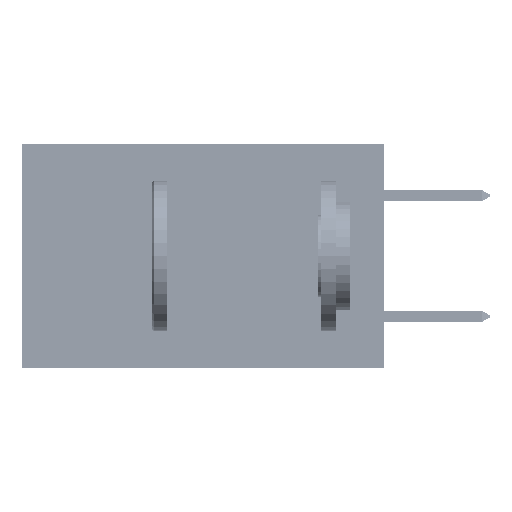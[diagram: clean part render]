
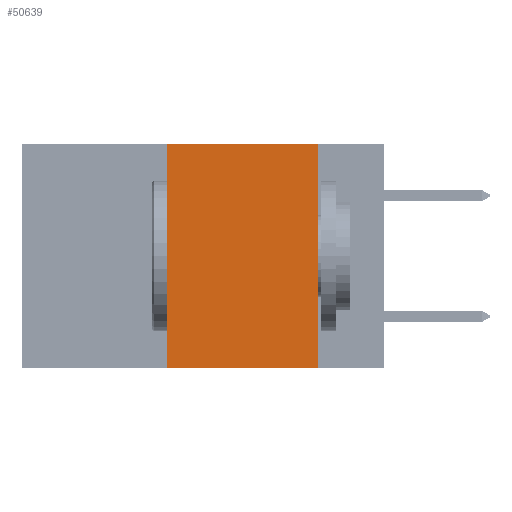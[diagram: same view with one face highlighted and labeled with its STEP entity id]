
A CAD part, left-side view. The second image highlights one B-rep face of the part: STEP entity #50639.
In plain terms, the highlighted planar face has unit normal (-1, 0, 0).
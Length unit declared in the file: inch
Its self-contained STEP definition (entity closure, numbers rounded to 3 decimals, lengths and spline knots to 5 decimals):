
#473 = VERTEX_POINT ( 'NONE', #18248 ) ;
#1398 = EDGE_LOOP ( 'NONE', ( #3842, #28397, #49163, #30030 ) ) ;
#3344 = VERTEX_POINT ( 'NONE', #49609 ) ;
#3842 = ORIENTED_EDGE ( 'NONE', *, *, #40647, .F. ) ;
#6336 = VECTOR ( 'NONE', #15519, 39.37008 ) ;
#7447 = LINE ( 'NONE', #50483, #43692 ) ;
#12015 = DIRECTION ( 'NONE',  ( 0., 0., -1. ) ) ;
#13848 = VERTEX_POINT ( 'NONE', #45142 ) ;
#13962 = AXIS2_PLACEMENT_3D ( 'NONE', #43008, #50385, #27043 ) ;
#15519 = DIRECTION ( 'NONE',  ( 0., -1., 0. ) ) ;
#17990 = LINE ( 'NONE', #35624, #6336 ) ;
#18248 = CARTESIAN_POINT ( 'NONE',  ( 0., 0.11, 0. ) ) ;
#19145 = PLANE ( 'NONE',  #13962 ) ;
#19431 = FACE_OUTER_BOUND ( 'NONE', #1398, .T. ) ;
#21513 = EDGE_CURVE ( 'NONE', #22364, #3344, #48150, .T. ) ;
#22288 = EDGE_CURVE ( 'NONE', #13848, #473, #17990, .T. ) ;
#22364 = VERTEX_POINT ( 'NONE', #38914 ) ;
#25880 = DIRECTION ( 'NONE',  ( 0., 0., 1. ) ) ;
#27043 = DIRECTION ( 'NONE',  ( 0., 0., -1. ) ) ;
#28397 = ORIENTED_EDGE ( 'NONE', *, *, #22288, .F. ) ;
#30030 = ORIENTED_EDGE ( 'NONE', *, *, #21513, .T. ) ;
#32541 = DIRECTION ( 'NONE',  ( 0., -1., 0. ) ) ;
#35624 = CARTESIAN_POINT ( 'NONE',  ( 0., 0.6, 0. ) ) ;
#35889 = EDGE_CURVE ( 'NONE', #22364, #13848, #7447, .T. ) ;
#37638 = LINE ( 'NONE', #43600, #43152 ) ;
#37717 = VECTOR ( 'NONE', #32541, 39.37008 ) ;
#38914 = CARTESIAN_POINT ( 'NONE',  ( 0., 0.36, -0.37 ) ) ;
#40647 = EDGE_CURVE ( 'NONE', #473, #3344, #37638, .T. ) ;
#43008 = CARTESIAN_POINT ( 'NONE',  ( 0., 0.6, 0. ) ) ;
#43152 = VECTOR ( 'NONE', #12015, 39.37008 ) ;
#43600 = CARTESIAN_POINT ( 'NONE',  ( 0., 0.11, 0. ) ) ;
#43692 = VECTOR ( 'NONE', #25880, 39.37008 ) ;
#45142 = CARTESIAN_POINT ( 'NONE',  ( 0., 0.36, 0. ) ) ;
#48150 = LINE ( 'NONE', #48354, #37717 ) ;
#48354 = CARTESIAN_POINT ( 'NONE',  ( 0., 0.6, -0.37 ) ) ;
#49163 = ORIENTED_EDGE ( 'NONE', *, *, #35889, .F. ) ;
#49609 = CARTESIAN_POINT ( 'NONE',  ( 0., 0.11, -0.37 ) ) ;
#50385 = DIRECTION ( 'NONE',  ( 1., 0., 0. ) ) ;
#50483 = CARTESIAN_POINT ( 'NONE',  ( 0., 0.36, 0. ) ) ;
#50639 = ADVANCED_FACE ( 'NONE', ( #19431 ), #19145, .F. ) ;
